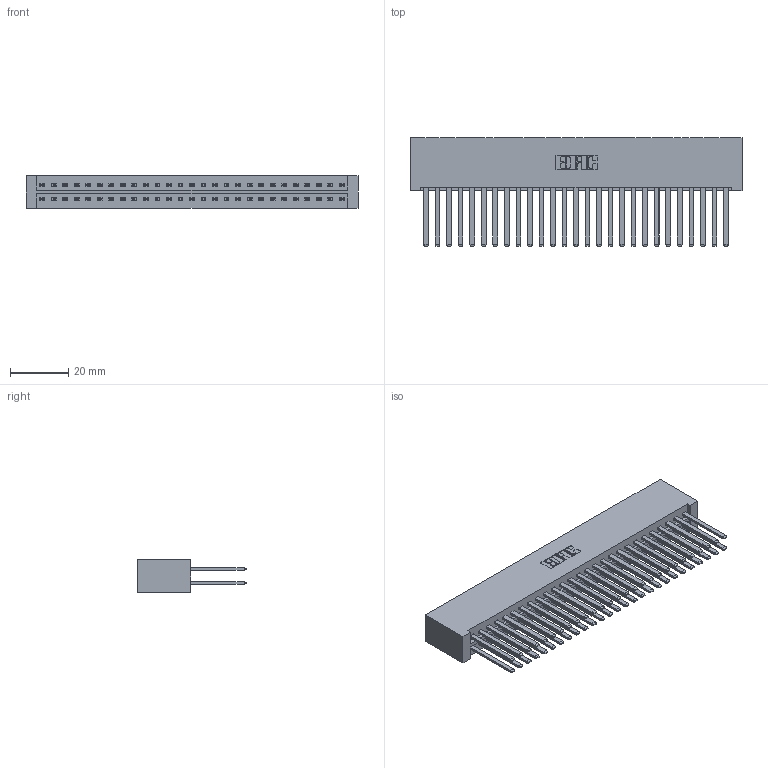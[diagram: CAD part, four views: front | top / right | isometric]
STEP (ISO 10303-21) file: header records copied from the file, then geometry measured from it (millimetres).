
FILE_DESCRIPTION (( 'STEP AP203' ), '1' );
FILE_NAME ('336-054-541-801.STEP', '2020-08-08T00:18:46', ( '' ), ( '' ), 'SwSTEP 2.0', 'SolidWorks 2020', '' );
FILE_SCHEMA (( 'CONFIG_CONTROL_DESIGN' ));
Length unit declared in the file: inch
Products named in the file (3): 336-290-001_336-290-541; 336-054-541-801; 336 Part_Lugless
Assembly tree (55 placements, depth 2):
  336-054-541-801
    336 Part_Lugless
    336-290-001_336-290-541  x54
Bounding box: 114.1 x 37.34 x 11.1 mm (x, y, z)
Volume: 18821.1 mm3; surface area: 23972.4 mm2
Topology: 55 solids, 55 shells, 2374 faces, 7145 edges, 4726 vertices
Faces by surface type: plane 1470, cylinder 904
Entity records: 22316 total; most frequent: CARTESIAN_POINT 3853, ORIENTED_EDGE 3690, DIRECTION 3201, EDGE_CURVE 1845, VECTOR 1721, LINE 1721, VERTEX_POINT 1228, AXIS2_PLACEMENT_3D 740
